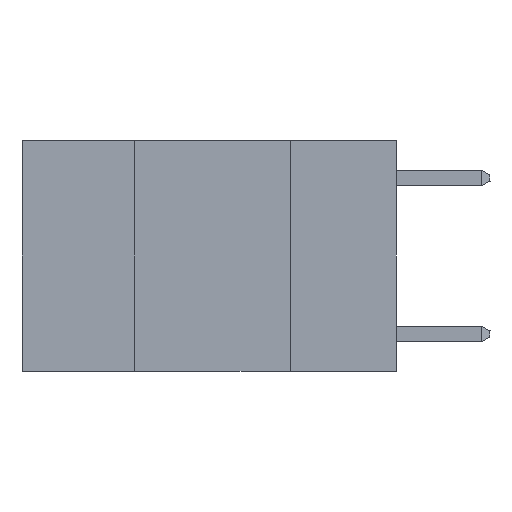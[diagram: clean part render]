
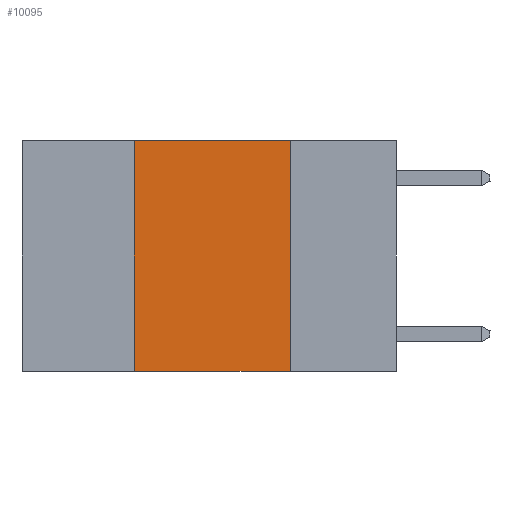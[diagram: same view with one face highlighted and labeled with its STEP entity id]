
A CAD part, left-side view. The second image highlights one B-rep face of the part: STEP entity #10095.
In plain terms, the highlighted planar face has unit normal (-1, 0, 0).
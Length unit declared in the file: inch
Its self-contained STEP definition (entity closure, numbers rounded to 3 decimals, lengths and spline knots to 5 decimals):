
#476 = VECTOR ( 'NONE', #18539, 39.37008 ) ;
#502 = CARTESIAN_POINT ( 'NONE',  ( 0., 0.17, 0. ) ) ;
#1958 = LINE ( 'NONE', #26965, #28496 ) ;
#1978 = CARTESIAN_POINT ( 'NONE',  ( 0., 0.6, 0. ) ) ;
#2111 = EDGE_CURVE ( 'NONE', #16420, #12551, #9624, .T. ) ;
#2455 = DIRECTION ( 'NONE',  ( 0., 0., 1. ) ) ;
#2846 = VECTOR ( 'NONE', #2455, 39.37008 ) ;
#3033 = LINE ( 'NONE', #21939, #4651 ) ;
#3537 = ORIENTED_EDGE ( 'NONE', *, *, #21760, .T. ) ;
#3573 = CARTESIAN_POINT ( 'NONE',  ( 0., 0.42, 0. ) ) ;
#3772 = ORIENTED_EDGE ( 'NONE', *, *, #2111, .F. ) ;
#3974 = DIRECTION ( 'NONE',  ( 0., 0., -1. ) ) ;
#4651 = VECTOR ( 'NONE', #26661, 39.37008 ) ;
#6406 = FACE_OUTER_BOUND ( 'NONE', #19951, .T. ) ;
#8654 = CARTESIAN_POINT ( 'NONE',  ( 0., 0.42, -0.37 ) ) ;
#9624 = LINE ( 'NONE', #18620, #2846 ) ;
#10095 = ADVANCED_FACE ( 'NONE', ( #6406 ), #27289, .F. ) ;
#12551 = VERTEX_POINT ( 'NONE', #3573 ) ;
#14760 = VERTEX_POINT ( 'NONE', #29890 ) ;
#15844 = DIRECTION ( 'NONE',  ( 0., 0., -1. ) ) ;
#16093 = LINE ( 'NONE', #22035, #476 ) ;
#16420 = VERTEX_POINT ( 'NONE', #8654 ) ;
#16709 = AXIS2_PLACEMENT_3D ( 'NONE', #1978, #30012, #3974 ) ;
#18539 = DIRECTION ( 'NONE',  ( 0., -1., 0. ) ) ;
#18620 = CARTESIAN_POINT ( 'NONE',  ( 0., 0.42, 0. ) ) ;
#19951 = EDGE_LOOP ( 'NONE', ( #22984, #20089, #3772, #3537 ) ) ;
#20089 = ORIENTED_EDGE ( 'NONE', *, *, #28131, .F. ) ;
#21760 = EDGE_CURVE ( 'NONE', #16420, #14760, #3033, .T. ) ;
#21939 = CARTESIAN_POINT ( 'NONE',  ( 0., 0.6, -0.37 ) ) ;
#22035 = CARTESIAN_POINT ( 'NONE',  ( 0., 0.6, 0. ) ) ;
#22984 = ORIENTED_EDGE ( 'NONE', *, *, #23206, .F. ) ;
#23206 = EDGE_CURVE ( 'NONE', #28782, #14760, #1958, .T. ) ;
#26661 = DIRECTION ( 'NONE',  ( 0., -1., 0. ) ) ;
#26965 = CARTESIAN_POINT ( 'NONE',  ( 0., 0.17, 0. ) ) ;
#27289 = PLANE ( 'NONE',  #16709 ) ;
#28131 = EDGE_CURVE ( 'NONE', #12551, #28782, #16093, .T. ) ;
#28496 = VECTOR ( 'NONE', #15844, 39.37008 ) ;
#28782 = VERTEX_POINT ( 'NONE', #502 ) ;
#29890 = CARTESIAN_POINT ( 'NONE',  ( 0., 0.17, -0.37 ) ) ;
#30012 = DIRECTION ( 'NONE',  ( 1., 0., 0. ) ) ;
